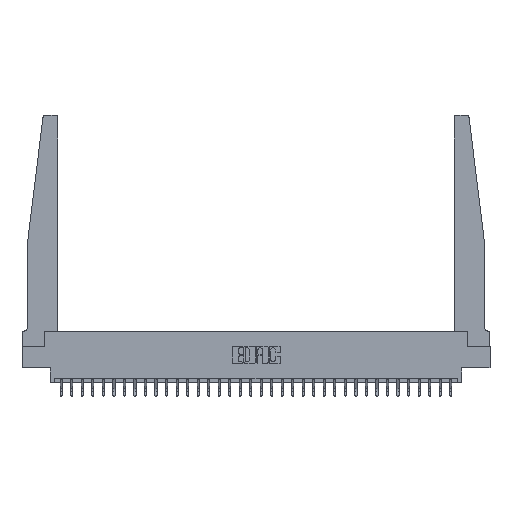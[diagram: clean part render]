
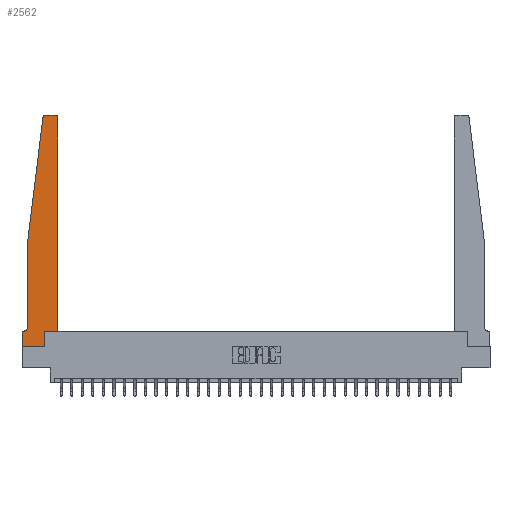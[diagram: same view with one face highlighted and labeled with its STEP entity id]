
A CAD part, top view. The second image highlights one B-rep face of the part: STEP entity #2562.
In plain terms, the highlighted planar face has unit normal (0, 0, 1).
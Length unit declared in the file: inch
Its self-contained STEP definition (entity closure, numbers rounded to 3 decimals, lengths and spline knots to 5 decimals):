
#112 = CARTESIAN_POINT ( 'NONE',  ( 0., 0., 0.37 ) ) ;
#119 = DIRECTION ( 'NONE',  ( 1., 0., 0. ) ) ;
#450 = CARTESIAN_POINT ( 'NONE',  ( 0.015, 0.2375, 0.37 ) ) ;
#575 = EDGE_CURVE ( 'NONE', #28473, #9293, #26944, .T. ) ;
#698 = PLANE ( 'NONE',  #1646 ) ;
#958 = CARTESIAN_POINT ( 'NONE',  ( 0.065, 0.2375, 0.37 ) ) ;
#973 = LINE ( 'NONE', #11510, #19027 ) ;
#1051 = ORIENTED_EDGE ( 'NONE', *, *, #575, .T. ) ;
#1242 = DIRECTION ( 'NONE',  ( 1., 0., 0. ) ) ;
#1646 = AXIS2_PLACEMENT_3D ( 'NONE', #21900, #12536, #29017 ) ;
#2482 = DIRECTION ( 'NONE',  ( 0., -1., 0. ) ) ;
#2562 = ADVANCED_FACE ( 'NONE', ( #3814 ), #698, .T. ) ;
#2814 = DIRECTION ( 'NONE',  ( -1., 0., 0. ) ) ;
#2822 = ORIENTED_EDGE ( 'NONE', *, *, #22598, .T. ) ;
#2897 = VECTOR ( 'NONE', #1242, 39.37008 ) ;
#3165 = VECTOR ( 'NONE', #24603, 39.37008 ) ;
#3250 = CARTESIAN_POINT ( 'NONE',  ( 0.395, 2.75, 0.37 ) ) ;
#3330 = CARTESIAN_POINT ( 'NONE',  ( 0.395, 2.72, 0.37 ) ) ;
#3814 = FACE_OUTER_BOUND ( 'NONE', #14520, .T. ) ;
#4839 = VERTEX_POINT ( 'NONE', #20569 ) ;
#5381 = ORIENTED_EDGE ( 'NONE', *, *, #27801, .T. ) ;
#5681 = DIRECTION ( 'NONE',  ( 1., 0., 0. ) ) ;
#5799 = VECTOR ( 'NONE', #14498, 39.37008 ) ;
#6071 = CARTESIAN_POINT ( 'NONE',  ( 0.24675, 2.72367, 0.37 ) ) ;
#6349 = EDGE_CURVE ( 'NONE', #4839, #28113, #23928, .T. ) ;
#6526 = ORIENTED_EDGE ( 'NONE', *, *, #17436, .T. ) ;
#6854 = EDGE_CURVE ( 'NONE', #9293, #28346, #23136, .T. ) ;
#7394 = VECTOR ( 'NONE', #27816, 39.37008 ) ;
#8179 = EDGE_CURVE ( 'NONE', #8189, #19402, #16414, .T. ) ;
#8189 = VERTEX_POINT ( 'NONE', #8231 ) ;
#8231 = CARTESIAN_POINT ( 'NONE',  ( 0.015, 0.1875, 0.37 ) ) ;
#8270 = CARTESIAN_POINT ( 'NONE',  ( 0.25, 2.75, 0.37 ) ) ;
#8505 = VERTEX_POINT ( 'NONE', #23450 ) ;
#8793 = EDGE_CURVE ( 'NONE', #8505, #28805, #11755, .T. ) ;
#8939 = VERTEX_POINT ( 'NONE', #20512 ) ;
#9152 = LINE ( 'NONE', #27113, #2897 ) ;
#9293 = VERTEX_POINT ( 'NONE', #12470 ) ;
#9789 = VECTOR ( 'NONE', #20091, 39.37008 ) ;
#11085 = EDGE_CURVE ( 'NONE', #28113, #8505, #973, .T. ) ;
#11510 = CARTESIAN_POINT ( 'NONE',  ( 0.425, 0.18, 0.37 ) ) ;
#11755 = CIRCLE ( 'NONE', #16931, 0.03 ) ;
#11892 = CARTESIAN_POINT ( 'NONE',  ( 0., 0., 0.37 ) ) ;
#11951 = EDGE_CURVE ( 'NONE', #28346, #8189, #23420, .T. ) ;
#12189 = DIRECTION ( 'NONE',  ( -0.122, -0.992, 0. ) ) ;
#12470 = CARTESIAN_POINT ( 'NONE',  ( 0.065, 1.25, 0.37 ) ) ;
#12536 = DIRECTION ( 'NONE',  ( 0., 0., 1. ) ) ;
#12863 = ORIENTED_EDGE ( 'NONE', *, *, #11085, .T. ) ;
#13639 = LINE ( 'NONE', #27721, #7394 ) ;
#13661 = VECTOR ( 'NONE', #12189, 39.37008 ) ;
#13868 = DIRECTION ( 'NONE',  ( 0., 1., 0. ) ) ;
#14120 = LINE ( 'NONE', #112, #25924 ) ;
#14226 = DIRECTION ( 'NONE',  ( 0., 0., 1. ) ) ;
#14498 = DIRECTION ( 'NONE',  ( 0., -1., 0. ) ) ;
#14520 = EDGE_LOOP ( 'NONE', ( #5381, #2822, #1051, #17646, #25473, #20810, #30389, #6526, #23142, #15128, #12863, #20608 ) ) ;
#15038 = CARTESIAN_POINT ( 'NONE',  ( 0.425, 0.18, 0.37 ) ) ;
#15128 = ORIENTED_EDGE ( 'NONE', *, *, #6349, .T. ) ;
#15218 = CARTESIAN_POINT ( 'NONE',  ( 0.065, 0.1875, 0.37 ) ) ;
#16414 = LINE ( 'NONE', #15218, #3165 ) ;
#16884 = VECTOR ( 'NONE', #17370, 39.37008 ) ;
#16902 = DIRECTION ( 'NONE',  ( 0., 0., -1. ) ) ;
#16931 = AXIS2_PLACEMENT_3D ( 'NONE', #3330, #19810, #5681 ) ;
#17370 = DIRECTION ( 'NONE',  ( 1., 0., 0. ) ) ;
#17436 = EDGE_CURVE ( 'NONE', #29961, #8939, #9152, .T. ) ;
#17646 = ORIENTED_EDGE ( 'NONE', *, *, #6854, .T. ) ;
#19027 = VECTOR ( 'NONE', #13868, 39.37008 ) ;
#19188 = AXIS2_PLACEMENT_3D ( 'NONE', #28333, #14226, #119 ) ;
#19402 = VERTEX_POINT ( 'NONE', #20604 ) ;
#19810 = DIRECTION ( 'NONE',  ( 0., 0., 1. ) ) ;
#20091 = DIRECTION ( 'NONE',  ( -1., 0., 0. ) ) ;
#20512 = CARTESIAN_POINT ( 'NONE',  ( 0.2605, 0., 0.37 ) ) ;
#20569 = CARTESIAN_POINT ( 'NONE',  ( 0.2605, 0.18, 0.37 ) ) ;
#20604 = CARTESIAN_POINT ( 'NONE',  ( 0., 0.1875, 0.37 ) ) ;
#20608 = ORIENTED_EDGE ( 'NONE', *, *, #8793, .T. ) ;
#20810 = ORIENTED_EDGE ( 'NONE', *, *, #8179, .T. ) ;
#21382 = EDGE_CURVE ( 'NONE', #19402, #29961, #14120, .T. ) ;
#21900 = CARTESIAN_POINT ( 'NONE',  ( 0., 0.1875, 0.37 ) ) ;
#22317 = LINE ( 'NONE', #8270, #9789 ) ;
#22598 = EDGE_CURVE ( 'NONE', #24678, #28473, #27022, .T. ) ;
#23136 = LINE ( 'NONE', #24299, #5799 ) ;
#23142 = ORIENTED_EDGE ( 'NONE', *, *, #28647, .T. ) ;
#23420 = CIRCLE ( 'NONE', #24326, 0.05 ) ;
#23450 = CARTESIAN_POINT ( 'NONE',  ( 0.425, 2.72, 0.37 ) ) ;
#23928 = LINE ( 'NONE', #15038, #16884 ) ;
#23952 = CARTESIAN_POINT ( 'NONE',  ( 0.065, 1.25, 0.37 ) ) ;
#24299 = CARTESIAN_POINT ( 'NONE',  ( 0.065, 1.25, 0.37 ) ) ;
#24326 = AXIS2_PLACEMENT_3D ( 'NONE', #450, #16902, #2814 ) ;
#24603 = DIRECTION ( 'NONE',  ( -1., 0., 0. ) ) ;
#24678 = VERTEX_POINT ( 'NONE', #26194 ) ;
#25473 = ORIENTED_EDGE ( 'NONE', *, *, #11951, .T. ) ;
#25850 = CARTESIAN_POINT ( 'NONE',  ( 0.425, 0.18, 0.37 ) ) ;
#25924 = VECTOR ( 'NONE', #2482, 39.37008 ) ;
#26194 = CARTESIAN_POINT ( 'NONE',  ( 0.27653, 2.75, 0.37 ) ) ;
#26944 = LINE ( 'NONE', #23952, #13661 ) ;
#27022 = CIRCLE ( 'NONE', #19188, 0.03 ) ;
#27113 = CARTESIAN_POINT ( 'NONE',  ( 0., 0., 0.37 ) ) ;
#27721 = CARTESIAN_POINT ( 'NONE',  ( 0.2605, 0.18, 0.37 ) ) ;
#27801 = EDGE_CURVE ( 'NONE', #28805, #24678, #22317, .T. ) ;
#27816 = DIRECTION ( 'NONE',  ( 0., 1., 0. ) ) ;
#28113 = VERTEX_POINT ( 'NONE', #25850 ) ;
#28333 = CARTESIAN_POINT ( 'NONE',  ( 0.27653, 2.72, 0.37 ) ) ;
#28346 = VERTEX_POINT ( 'NONE', #958 ) ;
#28473 = VERTEX_POINT ( 'NONE', #6071 ) ;
#28647 = EDGE_CURVE ( 'NONE', #8939, #4839, #13639, .T. ) ;
#28805 = VERTEX_POINT ( 'NONE', #3250 ) ;
#29017 = DIRECTION ( 'NONE',  ( 1., 0., 0. ) ) ;
#29961 = VERTEX_POINT ( 'NONE', #11892 ) ;
#30389 = ORIENTED_EDGE ( 'NONE', *, *, #21382, .T. ) ;
